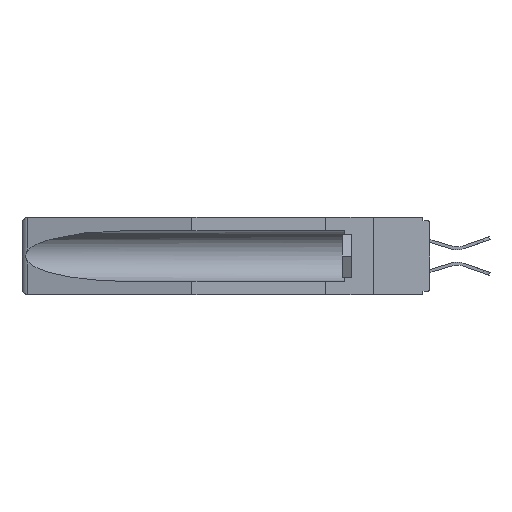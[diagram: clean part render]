
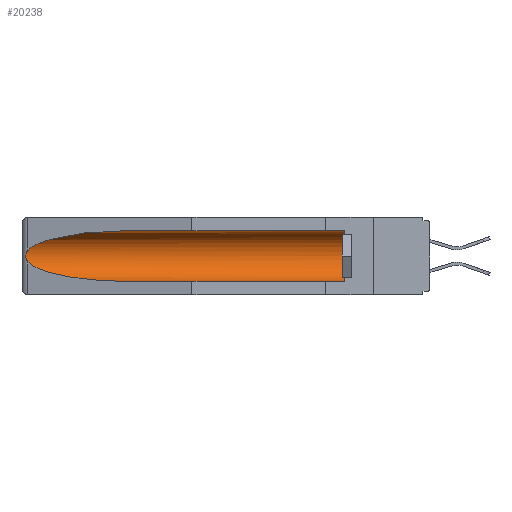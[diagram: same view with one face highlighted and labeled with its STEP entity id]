
A CAD part, left-side view. The second image highlights one B-rep face of the part: STEP entity #20238.
In plain terms, the highlighted cylindrical face has radius 2.857 mm (diameter 5.715 mm), a partial arc.
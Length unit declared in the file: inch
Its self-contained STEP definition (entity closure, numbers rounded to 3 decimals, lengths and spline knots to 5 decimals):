
#259 = CARTESIAN_POINT ( 'NONE',  ( 0.155, 1.07973, -0.059 ) ) ;
#964 = CARTESIAN_POINT ( 'NONE',  ( 0.21114, 1.30732, -0.284 ) ) ;
#2123 = CARTESIAN_POINT ( 'NONE',  ( 0.25451, 1.48313, -0.09465 ) ) ;
#2226 = CARTESIAN_POINT ( 'NONE',  ( 0.155, 0.126, -0.284 ) ) ;
#2638 = DIRECTION ( 'NONE',  ( 0., 1., 0. ) ) ;
#2760 = VERTEX_POINT ( 'NONE', #14543 ) ;
#3874 = CARTESIAN_POINT ( 'NONE',  ( 0.155, 0.126, -0.1715 ) ) ;
#4037 = EDGE_LOOP ( 'NONE', ( #16958, #26128, #14319, #15165, #20757, #5348 ) ) ;
#5348 = ORIENTED_EDGE ( 'NONE', *, *, #24577, .T. ) ;
#5661 = EDGE_CURVE ( 'NONE', #18730, #20748, #16847, .T. ) ;
#5696 = LINE ( 'NONE', #11356, #11349 ) ;
#5802 =( BOUNDED_CURVE ( )  B_SPLINE_CURVE ( 3, ( #259, #15690, #2123, #13595 ),
 .UNSPECIFIED., .F., .F. ) 
 B_SPLINE_CURVE_WITH_KNOTS ( ( 4, 4 ),
 ( 4.71239, 6.08839 ),
 .UNSPECIFIED. ) 
 CURVE ( )  GEOMETRIC_REPRESENTATION_ITEM ( )  RATIONAL_B_SPLINE_CURVE ( ( 1., 0.848, 0.848, 1. ) ) 
 REPRESENTATION_ITEM ( '' )  );
#7175 = CARTESIAN_POINT ( 'NONE',  ( 0.155, -0.30754, -0.284 ) ) ;
#8074 = CARTESIAN_POINT ( 'NONE',  ( 0.26654, 1.53092, -0.15636 ) ) ;
#8290 = DIRECTION ( 'NONE',  ( 0., -1., 0. ) ) ;
#9980 = EDGE_CURVE ( 'NONE', #17588, #2760, #15722, .T. ) ;
#10131 = CARTESIAN_POINT ( 'NONE',  ( 0.2675, 1.53308, -0.17534 ) ) ;
#10233 = CARTESIAN_POINT ( 'NONE',  ( 0.26597, 1.52961, -0.15275 ) ) ;
#10383 = EDGE_CURVE ( 'NONE', #13827, #18730, #19014, .T. ) ;
#10842 = LINE ( 'NONE', #7175, #21131 ) ;
#11349 = VECTOR ( 'NONE', #15733, 39.37008 ) ;
#11356 = CARTESIAN_POINT ( 'NONE',  ( 0.155, -0.30754, -0.059 ) ) ;
#13595 = CARTESIAN_POINT ( 'NONE',  ( 0.26537, 1.52718, -0.14972 ) ) ;
#13827 = VERTEX_POINT ( 'NONE', #21613 ) ;
#14319 = ORIENTED_EDGE ( 'NONE', *, *, #5661, .T. ) ;
#14501 = CARTESIAN_POINT ( 'NONE',  ( 0.26597, 1.5296, -0.19026 ) ) ;
#14543 = CARTESIAN_POINT ( 'NONE',  ( 0.155, 0.126, -0.059 ) ) ;
#14603 = CARTESIAN_POINT ( 'NONE',  ( 0.26537, 1.52718, -0.19328 ) ) ;
#14605 = CARTESIAN_POINT ( 'NONE',  ( 0.155, 1.07973, -0.059 ) ) ;
#14660 = CARTESIAN_POINT ( 'NONE',  ( 0.155, 1.07973, -0.284 ) ) ;
#14697 = CARTESIAN_POINT ( 'NONE',  ( 0.26537, 1.52718, -0.14972 ) ) ;
#14725 = AXIS2_PLACEMENT_3D ( 'NONE', #3874, #8290, #24063 ) ;
#15165 = ORIENTED_EDGE ( 'NONE', *, *, #19806, .F. ) ;
#15690 = CARTESIAN_POINT ( 'NONE',  ( 0.21114, 1.30732, -0.059 ) ) ;
#15722 = CIRCLE ( 'NONE', #14725, 0.1125 ) ;
#15733 = DIRECTION ( 'NONE',  ( 0., 1., 0. ) ) ;
#16847 =( BOUNDED_CURVE ( )  B_SPLINE_CURVE ( 3, ( #28498, #28401, #964, #21433 ),
 .UNSPECIFIED., .F., .F. ) 
 B_SPLINE_CURVE_WITH_KNOTS ( ( 4, 4 ),
 ( 0.1948, 1.5708 ),
 .UNSPECIFIED. ) 
 CURVE ( )  GEOMETRIC_REPRESENTATION_ITEM ( )  RATIONAL_B_SPLINE_CURVE ( ( 1., 0.848, 0.848, 1. ) ) 
 REPRESENTATION_ITEM ( '' )  );
#16892 = CARTESIAN_POINT ( 'NONE',  ( 0.26655, 1.53094, -0.18657 ) ) ;
#16958 = ORIENTED_EDGE ( 'NONE', *, *, #26344, .T. ) ;
#17588 = VERTEX_POINT ( 'NONE', #2226 ) ;
#18612 = CYLINDRICAL_SURFACE ( 'NONE', #23511, 0.1125 ) ;
#18730 = VERTEX_POINT ( 'NONE', #21806 ) ;
#19014 = B_SPLINE_CURVE_WITH_KNOTS ( 'NONE', 3,
 ( #14697, #10233, #8074, #23851, #28014, #10131, #19252, #16892, #14501, #14603 ),
 .UNSPECIFIED., .F., .F.,
 ( 4, 2, 2, 2, 4 ),
 ( 0., 0.00029, 0.00058, 0.00087, 0.00117 ),
 .UNSPECIFIED. ) ;
#19252 = CARTESIAN_POINT ( 'NONE',  ( 0.2673, 1.53269, -0.17917 ) ) ;
#19806 = EDGE_CURVE ( 'NONE', #17588, #20748, #10842, .T. ) ;
#20034 = FACE_OUTER_BOUND ( 'NONE', #4037, .T. ) ;
#20238 = ADVANCED_FACE ( 'NONE', ( #20034 ), #18612, .F. ) ;
#20748 = VERTEX_POINT ( 'NONE', #14660 ) ;
#20757 = ORIENTED_EDGE ( 'NONE', *, *, #9980, .T. ) ;
#21131 = VECTOR ( 'NONE', #2638, 39.37008 ) ;
#21134 = DIRECTION ( 'NONE',  ( 0., 1., 0. ) ) ;
#21433 = CARTESIAN_POINT ( 'NONE',  ( 0.155, 1.07973, -0.284 ) ) ;
#21613 = CARTESIAN_POINT ( 'NONE',  ( 0.26537, 1.52718, -0.14972 ) ) ;
#21806 = CARTESIAN_POINT ( 'NONE',  ( 0.26537, 1.52718, -0.19328 ) ) ;
#23511 = AXIS2_PLACEMENT_3D ( 'NONE', #25819, #21134, #23645 ) ;
#23645 = DIRECTION ( 'NONE',  ( 0., 0., 1. ) ) ;
#23851 = CARTESIAN_POINT ( 'NONE',  ( 0.2673, 1.5327, -0.16383 ) ) ;
#24063 = DIRECTION ( 'NONE',  ( 0., 0., 1. ) ) ;
#24577 = EDGE_CURVE ( 'NONE', #2760, #27758, #5696, .T. ) ;
#25819 = CARTESIAN_POINT ( 'NONE',  ( 0.155, -0.30754, -0.1715 ) ) ;
#26128 = ORIENTED_EDGE ( 'NONE', *, *, #10383, .T. ) ;
#26344 = EDGE_CURVE ( 'NONE', #27758, #13827, #5802, .T. ) ;
#27758 = VERTEX_POINT ( 'NONE', #14605 ) ;
#28014 = CARTESIAN_POINT ( 'NONE',  ( 0.2675, 1.53308, -0.16763 ) ) ;
#28401 = CARTESIAN_POINT ( 'NONE',  ( 0.25451, 1.48313, -0.24835 ) ) ;
#28498 = CARTESIAN_POINT ( 'NONE',  ( 0.26537, 1.52718, -0.19328 ) ) ;
